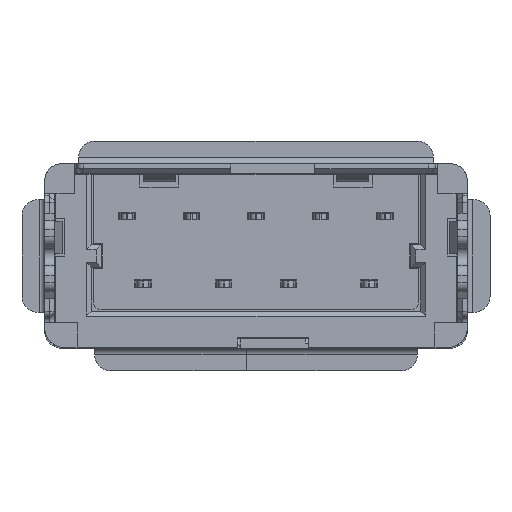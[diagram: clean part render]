
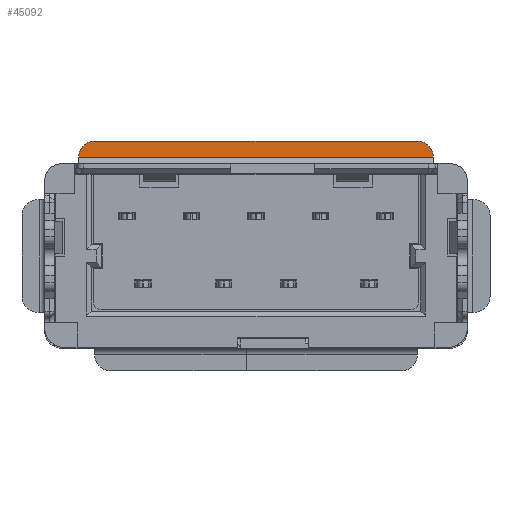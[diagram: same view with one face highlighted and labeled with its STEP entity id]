
A CAD part, front view. The second image highlights one B-rep face of the part: STEP entity #45092.
In plain terms, the highlighted face is planar.
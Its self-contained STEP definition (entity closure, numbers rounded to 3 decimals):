
#1322 = DIRECTION ( 'NONE',  ( -1., 0., 0. ) ) ;
#3635 = ORIENTED_EDGE ( 'NONE', *, *, #36679, .F. ) ;
#4262 = VECTOR ( 'NONE', #25280, 1000. ) ;
#5143 = CARTESIAN_POINT ( 'NONE',  ( 0., -10.18, -3.06 ) ) ;
#5386 = LINE ( 'NONE', #5143, #26233 ) ;
#7311 = EDGE_CURVE ( 'NONE', #11128, #23572, #5386, .T. ) ;
#7724 = VERTEX_POINT ( 'NONE', #41760 ) ;
#9361 = DIRECTION ( 'NONE',  ( 0., 1., 0. ) ) ;
#11128 = VERTEX_POINT ( 'NONE', #30806 ) ;
#11210 = EDGE_CURVE ( 'NONE', #11128, #36528, #34988, .T. ) ;
#11372 = DIRECTION ( 'NONE',  ( 0., -1., 0. ) ) ;
#14796 = EDGE_CURVE ( 'NONE', #7724, #23572, #37151, .T. ) ;
#15067 = ORIENTED_EDGE ( 'NONE', *, *, #11210, .T. ) ;
#16511 = DIRECTION ( 'NONE',  ( 0., 0., -1. ) ) ;
#16685 = ORIENTED_EDGE ( 'NONE', *, *, #7311, .F. ) ;
#17383 = AXIS2_PLACEMENT_3D ( 'NONE', #28272, #35190, #42571 ) ;
#17898 = LINE ( 'NONE', #28868, #4262 ) ;
#20889 = AXIS2_PLACEMENT_3D ( 'NONE', #44005, #11372, #22314 ) ;
#22314 = DIRECTION ( 'NONE',  ( 1., 0., 0. ) ) ;
#22583 = CARTESIAN_POINT ( 'NONE',  ( -5.5, -10.18, -3.06 ) ) ;
#23572 = VERTEX_POINT ( 'NONE', #22583 ) ;
#25140 = EDGE_LOOP ( 'NONE', ( #16685, #15067, #3635, #40456 ) ) ;
#25280 = DIRECTION ( 'NONE',  ( 1., 0., 0. ) ) ;
#26233 = VECTOR ( 'NONE', #1322, 1000. ) ;
#28272 = CARTESIAN_POINT ( 'NONE',  ( -5., -10.18, -3.06 ) ) ;
#28868 = CARTESIAN_POINT ( 'NONE',  ( 0., -10.18, -3.56 ) ) ;
#29240 = FACE_OUTER_BOUND ( 'NONE', #25140, .T. ) ;
#30806 = CARTESIAN_POINT ( 'NONE',  ( 5.5, -10.18, -3.06 ) ) ;
#33751 = PLANE ( 'NONE',  #20889 ) ;
#34988 = CIRCLE ( 'NONE', #41843, 0.5 ) ;
#35190 = DIRECTION ( 'NONE',  ( 0., 1., 0. ) ) ;
#36528 = VERTEX_POINT ( 'NONE', #39340 ) ;
#36679 = EDGE_CURVE ( 'NONE', #7724, #36528, #17898, .T. ) ;
#37151 = CIRCLE ( 'NONE', #17383, 0.5 ) ;
#39340 = CARTESIAN_POINT ( 'NONE',  ( 5., -10.18, -3.56 ) ) ;
#40456 = ORIENTED_EDGE ( 'NONE', *, *, #14796, .T. ) ;
#41760 = CARTESIAN_POINT ( 'NONE',  ( -5., -10.18, -3.56 ) ) ;
#41843 = AXIS2_PLACEMENT_3D ( 'NONE', #45779, #9361, #16511 ) ;
#42571 = DIRECTION ( 'NONE',  ( 0., 0., -1. ) ) ;
#44005 = CARTESIAN_POINT ( 'NONE',  ( -5.72, -10.18, -3.589 ) ) ;
#45092 = ADVANCED_FACE ( 'NONE', ( #29240 ), #33751, .F. ) ;
#45779 = CARTESIAN_POINT ( 'NONE',  ( 5., -10.18, -3.06 ) ) ;
